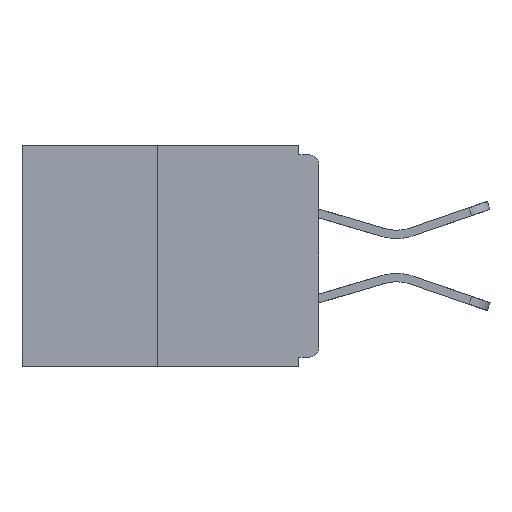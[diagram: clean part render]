
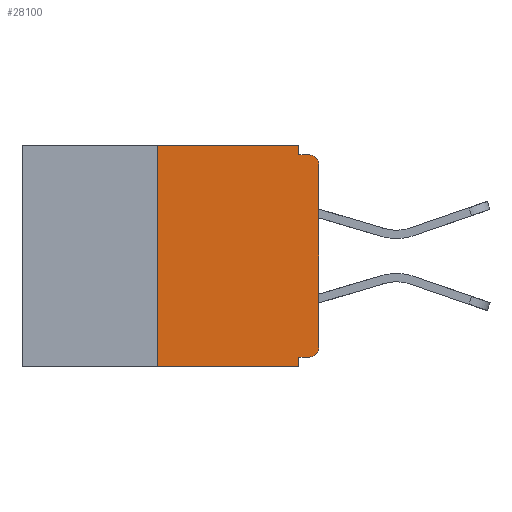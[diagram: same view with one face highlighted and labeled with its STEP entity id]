
A CAD part, left-side view. The second image highlights one B-rep face of the part: STEP entity #28100.
In plain terms, the highlighted planar face has unit normal (-1, 0, 0).
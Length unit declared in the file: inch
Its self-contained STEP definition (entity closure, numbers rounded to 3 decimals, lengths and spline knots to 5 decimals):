
#117 = CARTESIAN_POINT ( 'NONE',  ( 0., 0.015, -0.313 ) ) ;
#452 = DIRECTION ( 'NONE',  ( -1., 0., 0. ) ) ;
#605 = DIRECTION ( 'NONE',  ( 0., 0., -1. ) ) ;
#1206 = VERTEX_POINT ( 'NONE', #15921 ) ;
#1275 = LINE ( 'NONE', #20788, #8561 ) ;
#1448 = CARTESIAN_POINT ( 'NONE',  ( 0., 0.46, -0.343 ) ) ;
#1913 = CIRCLE ( 'NONE', #7655, 0.015 ) ;
#1959 = FACE_OUTER_BOUND ( 'NONE', #22554, .T. ) ;
#2367 = EDGE_CURVE ( 'NONE', #24105, #1206, #4762, .T. ) ;
#2470 = DIRECTION ( 'NONE',  ( 0., 0., -1. ) ) ;
#2610 = CARTESIAN_POINT ( 'NONE',  ( 0., 0., -0.313 ) ) ;
#3150 = AXIS2_PLACEMENT_3D ( 'NONE', #11858, #21933, #22577 ) ;
#3280 = EDGE_CURVE ( 'NONE', #28713, #11589, #29893, .T. ) ;
#3434 = VECTOR ( 'NONE', #2470, 39.37008 ) ;
#3690 = VERTEX_POINT ( 'NONE', #7748 ) ;
#4196 = CARTESIAN_POINT ( 'NONE',  ( 0., 0.031, -0.343 ) ) ;
#4762 = LINE ( 'NONE', #19706, #31240 ) ;
#4992 = VECTOR ( 'NONE', #18357, 39.37008 ) ;
#5044 = DIRECTION ( 'NONE',  ( 0., 0., 1. ) ) ;
#5215 = EDGE_CURVE ( 'NONE', #28713, #28463, #9074, .T. ) ;
#7100 = ORIENTED_EDGE ( 'NONE', *, *, #12781, .F. ) ;
#7655 = AXIS2_PLACEMENT_3D ( 'NONE', #117, #10206, #30039 ) ;
#7748 = CARTESIAN_POINT ( 'NONE',  ( 0., 0.031, -0.328 ) ) ;
#8271 = EDGE_CURVE ( 'NONE', #23881, #3690, #1275, .T. ) ;
#8458 = ORIENTED_EDGE ( 'NONE', *, *, #2367, .F. ) ;
#8500 = VECTOR ( 'NONE', #5044, 39.37008 ) ;
#8561 = VECTOR ( 'NONE', #20630, 39.37008 ) ;
#8929 = LINE ( 'NONE', #23554, #4992 ) ;
#9058 = ORIENTED_EDGE ( 'NONE', *, *, #21582, .T. ) ;
#9074 = LINE ( 'NONE', #1448, #18650 ) ;
#9943 = ORIENTED_EDGE ( 'NONE', *, *, #21540, .F. ) ;
#9989 = VECTOR ( 'NONE', #24681, 39.37008 ) ;
#10206 = DIRECTION ( 'NONE',  ( -1., 0., 0. ) ) ;
#11589 = VERTEX_POINT ( 'NONE', #14102 ) ;
#11776 = CARTESIAN_POINT ( 'NONE',  ( 0., 0., -0.03 ) ) ;
#11858 = CARTESIAN_POINT ( 'NONE',  ( 0., 0.46, 0. ) ) ;
#12658 = CARTESIAN_POINT ( 'NONE',  ( 0., 0., 0. ) ) ;
#12781 = EDGE_CURVE ( 'NONE', #11589, #14800, #8929, .T. ) ;
#14102 = CARTESIAN_POINT ( 'NONE',  ( 0., 0.25, 0. ) ) ;
#14799 = LINE ( 'NONE', #24720, #3434 ) ;
#14800 = VERTEX_POINT ( 'NONE', #26892 ) ;
#15196 = ORIENTED_EDGE ( 'NONE', *, *, #5215, .T. ) ;
#15238 = CARTESIAN_POINT ( 'NONE',  ( 0., 0.25, 0. ) ) ;
#15921 = CARTESIAN_POINT ( 'NONE',  ( 0., 0.015, -0.015 ) ) ;
#16776 = EDGE_CURVE ( 'NONE', #16824, #20440, #22272, .T. ) ;
#16824 = VERTEX_POINT ( 'NONE', #2610 ) ;
#18357 = DIRECTION ( 'NONE',  ( 0., -1., 0. ) ) ;
#18650 = VECTOR ( 'NONE', #26460, 39.37008 ) ;
#19706 = CARTESIAN_POINT ( 'NONE',  ( 0., 0., -0.015 ) ) ;
#20440 = VERTEX_POINT ( 'NONE', #11776 ) ;
#20630 = DIRECTION ( 'NONE',  ( 0., 1., 0. ) ) ;
#20788 = CARTESIAN_POINT ( 'NONE',  ( 0., 0., -0.328 ) ) ;
#21540 = EDGE_CURVE ( 'NONE', #3690, #28463, #25309, .T. ) ;
#21582 = EDGE_CURVE ( 'NONE', #23881, #16824, #1913, .T. ) ;
#21933 = DIRECTION ( 'NONE',  ( 1., 0., 0. ) ) ;
#22208 = ORIENTED_EDGE ( 'NONE', *, *, #23211, .F. ) ;
#22272 = LINE ( 'NONE', #12658, #8500 ) ;
#22554 = EDGE_LOOP ( 'NONE', ( #7100, #24025, #15196, #9943, #31006, #9058, #23754, #23043, #8458, #22208 ) ) ;
#22577 = DIRECTION ( 'NONE',  ( 0., 0., -1. ) ) ;
#22877 = CARTESIAN_POINT ( 'NONE',  ( 0., 0.031, -0.343 ) ) ;
#23018 = CARTESIAN_POINT ( 'NONE',  ( 0., 0.25, -0.343 ) ) ;
#23043 = ORIENTED_EDGE ( 'NONE', *, *, #23788, .T. ) ;
#23211 = EDGE_CURVE ( 'NONE', #14800, #24105, #14799, .T. ) ;
#23554 = CARTESIAN_POINT ( 'NONE',  ( 0., 0.46, 0. ) ) ;
#23754 = ORIENTED_EDGE ( 'NONE', *, *, #16776, .T. ) ;
#23788 = EDGE_CURVE ( 'NONE', #20440, #1206, #25762, .T. ) ;
#23881 = VERTEX_POINT ( 'NONE', #31465 ) ;
#24025 = ORIENTED_EDGE ( 'NONE', *, *, #3280, .F. ) ;
#24105 = VERTEX_POINT ( 'NONE', #25106 ) ;
#24681 = DIRECTION ( 'NONE',  ( 0., 0., 1. ) ) ;
#24720 = CARTESIAN_POINT ( 'NONE',  ( 0., 0.031, 0. ) ) ;
#25106 = CARTESIAN_POINT ( 'NONE',  ( 0., 0.031, -0.015 ) ) ;
#25309 = LINE ( 'NONE', #22877, #29443 ) ;
#25762 = CIRCLE ( 'NONE', #28872, 0.015 ) ;
#26162 = PLANE ( 'NONE',  #3150 ) ;
#26460 = DIRECTION ( 'NONE',  ( 0., -1., 0. ) ) ;
#26892 = CARTESIAN_POINT ( 'NONE',  ( 0., 0.031, 0. ) ) ;
#27932 = CARTESIAN_POINT ( 'NONE',  ( 0., 0.015, -0.03 ) ) ;
#28100 = ADVANCED_FACE ( 'NONE', ( #1959 ), #26162, .F. ) ;
#28463 = VERTEX_POINT ( 'NONE', #4196 ) ;
#28713 = VERTEX_POINT ( 'NONE', #23018 ) ;
#28872 = AXIS2_PLACEMENT_3D ( 'NONE', #27932, #452, #30214 ) ;
#29443 = VECTOR ( 'NONE', #605, 39.37008 ) ;
#29640 = DIRECTION ( 'NONE',  ( 0., -1., 0. ) ) ;
#29893 = LINE ( 'NONE', #15238, #9989 ) ;
#30039 = DIRECTION ( 'NONE',  ( 0., 0., -1. ) ) ;
#30214 = DIRECTION ( 'NONE',  ( 0., 0., -1. ) ) ;
#31006 = ORIENTED_EDGE ( 'NONE', *, *, #8271, .F. ) ;
#31240 = VECTOR ( 'NONE', #29640, 39.37008 ) ;
#31465 = CARTESIAN_POINT ( 'NONE',  ( 0., 0.015, -0.328 ) ) ;
